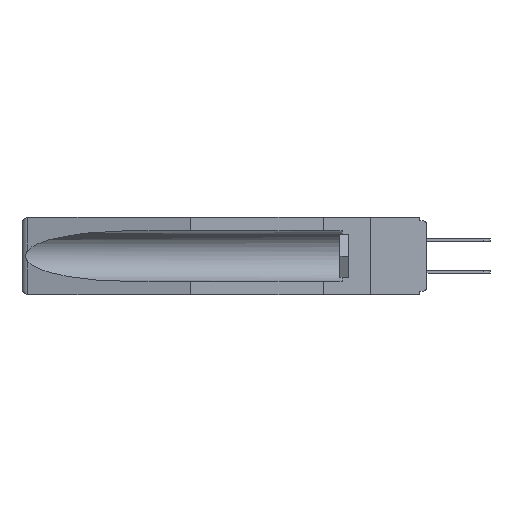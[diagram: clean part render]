
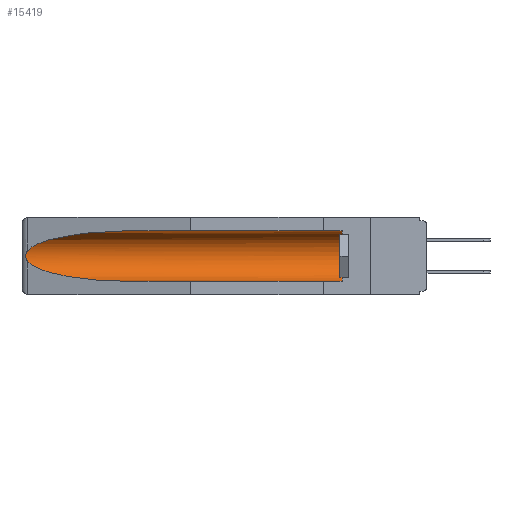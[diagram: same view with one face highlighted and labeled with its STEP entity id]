
A CAD part, left-side view. The second image highlights one B-rep face of the part: STEP entity #15419.
In plain terms, the highlighted cylindrical face has radius 2.857 mm (diameter 5.715 mm), a partial arc.
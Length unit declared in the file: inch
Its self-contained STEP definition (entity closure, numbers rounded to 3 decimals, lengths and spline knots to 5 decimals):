
#138 = CARTESIAN_POINT ( 'NONE',  ( 0.26654, 1.53092, -0.15636 ) ) ;
#239 = VECTOR ( 'NONE', #20241, 39.37008 ) ;
#244 = DIRECTION ( 'NONE',  ( 0., 1., 0. ) ) ;
#271 = CARTESIAN_POINT ( 'NONE',  ( 0.26537, 1.52718, -0.19328 ) ) ;
#353 = CARTESIAN_POINT ( 'NONE',  ( 0.26597, 1.5296, -0.19026 ) ) ;
#610 = ORIENTED_EDGE ( 'NONE', *, *, #13856, .T. ) ;
#1701 = ORIENTED_EDGE ( 'NONE', *, *, #15027, .T. ) ;
#2246 = CARTESIAN_POINT ( 'NONE',  ( 0.155, 1.07973, -0.284 ) ) ;
#2735 = DIRECTION ( 'NONE',  ( 0., 0., 1. ) ) ;
#3331 = VECTOR ( 'NONE', #244, 39.37008 ) ;
#3438 = CARTESIAN_POINT ( 'NONE',  ( 0.2675, 1.53308, -0.17534 ) ) ;
#3753 = ORIENTED_EDGE ( 'NONE', *, *, #21781, .T. ) ;
#3792 = AXIS2_PLACEMENT_3D ( 'NONE', #18318, #21011, #2735 ) ;
#4294 = EDGE_CURVE ( 'NONE', #19812, #9794, #5132, .T. ) ;
#4777 = CARTESIAN_POINT ( 'NONE',  ( 0.21114, 1.30732, -0.284 ) ) ;
#5132 = B_SPLINE_CURVE_WITH_KNOTS ( 'NONE', 3,
 ( #18709, #20573, #138, #10422, #12054, #3438, #15374, #8821, #353, #271 ),
 .UNSPECIFIED., .F., .F.,
 ( 4, 2, 2, 2, 4 ),
 ( 0., 0.00029, 0.00058, 0.00087, 0.00117 ),
 .UNSPECIFIED. ) ;
#5380 = EDGE_CURVE ( 'NONE', #13100, #5696, #18282, .T. ) ;
#5520 = CARTESIAN_POINT ( 'NONE',  ( 0.155, 0.126, -0.059 ) ) ;
#5696 = VERTEX_POINT ( 'NONE', #20296 ) ;
#6453 = AXIS2_PLACEMENT_3D ( 'NONE', #6814, #18595, #10385 ) ;
#6814 = CARTESIAN_POINT ( 'NONE',  ( 0.155, 0.126, -0.1715 ) ) ;
#6970 = CYLINDRICAL_SURFACE ( 'NONE', #3792, 0.1125 ) ;
#7698 = ORIENTED_EDGE ( 'NONE', *, *, #19265, .F. ) ;
#8676 = CARTESIAN_POINT ( 'NONE',  ( 0.26537, 1.52718, -0.19328 ) ) ;
#8821 = CARTESIAN_POINT ( 'NONE',  ( 0.26655, 1.53094, -0.18657 ) ) ;
#8995 = CARTESIAN_POINT ( 'NONE',  ( 0.26537, 1.52718, -0.14972 ) ) ;
#9185 = CARTESIAN_POINT ( 'NONE',  ( 0.26537, 1.52718, -0.14972 ) ) ;
#9591 = CARTESIAN_POINT ( 'NONE',  ( 0.155, 1.07973, -0.284 ) ) ;
#9794 = VERTEX_POINT ( 'NONE', #8676 ) ;
#9878 = VERTEX_POINT ( 'NONE', #2246 ) ;
#10385 = DIRECTION ( 'NONE',  ( 0., 0., 1. ) ) ;
#10422 = CARTESIAN_POINT ( 'NONE',  ( 0.2673, 1.5327, -0.16383 ) ) ;
#10460 = CARTESIAN_POINT ( 'NONE',  ( 0.155, -0.30754, -0.284 ) ) ;
#11533 = CARTESIAN_POINT ( 'NONE',  ( 0.26537, 1.52718, -0.19328 ) ) ;
#12054 = CARTESIAN_POINT ( 'NONE',  ( 0.2675, 1.53308, -0.16763 ) ) ;
#12168 = CARTESIAN_POINT ( 'NONE',  ( 0.21114, 1.30732, -0.059 ) ) ;
#13100 = VERTEX_POINT ( 'NONE', #5520 ) ;
#13334 = CARTESIAN_POINT ( 'NONE',  ( 0.155, -0.30754, -0.059 ) ) ;
#13683 = ORIENTED_EDGE ( 'NONE', *, *, #5380, .T. ) ;
#13729 = EDGE_LOOP ( 'NONE', ( #1701, #15863, #3753, #7698, #610, #13683 ) ) ;
#13856 = EDGE_CURVE ( 'NONE', #19405, #13100, #14693, .T. ) ;
#14103 = FACE_OUTER_BOUND ( 'NONE', #13729, .T. ) ;
#14693 = CIRCLE ( 'NONE', #6453, 0.1125 ) ;
#14937 = CARTESIAN_POINT ( 'NONE',  ( 0.25451, 1.48313, -0.24835 ) ) ;
#15027 = EDGE_CURVE ( 'NONE', #5696, #19812, #21580, .T. ) ;
#15374 = CARTESIAN_POINT ( 'NONE',  ( 0.2673, 1.53269, -0.17917 ) ) ;
#15419 = ADVANCED_FACE ( 'NONE', ( #14103 ), #6970, .F. ) ;
#15626 = CARTESIAN_POINT ( 'NONE',  ( 0.25451, 1.48313, -0.09465 ) ) ;
#15751 = CARTESIAN_POINT ( 'NONE',  ( 0.155, 1.07973, -0.059 ) ) ;
#15863 = ORIENTED_EDGE ( 'NONE', *, *, #4294, .T. ) ;
#18182 = CARTESIAN_POINT ( 'NONE',  ( 0.155, 0.126, -0.284 ) ) ;
#18282 = LINE ( 'NONE', #13334, #239 ) ;
#18318 = CARTESIAN_POINT ( 'NONE',  ( 0.155, -0.30754, -0.1715 ) ) ;
#18595 = DIRECTION ( 'NONE',  ( 0., -1., 0. ) ) ;
#18709 = CARTESIAN_POINT ( 'NONE',  ( 0.26537, 1.52718, -0.14972 ) ) ;
#19257 =( BOUNDED_CURVE ( )  B_SPLINE_CURVE ( 3, ( #11533, #14937, #4777, #9591 ),
 .UNSPECIFIED., .F., .F. ) 
 B_SPLINE_CURVE_WITH_KNOTS ( ( 4, 4 ),
 ( 0.1948, 1.5708 ),
 .UNSPECIFIED. ) 
 CURVE ( )  GEOMETRIC_REPRESENTATION_ITEM ( )  RATIONAL_B_SPLINE_CURVE ( ( 1., 0.848, 0.848, 1. ) ) 
 REPRESENTATION_ITEM ( '' )  );
#19265 = EDGE_CURVE ( 'NONE', #19405, #9878, #20850, .T. ) ;
#19405 = VERTEX_POINT ( 'NONE', #18182 ) ;
#19812 = VERTEX_POINT ( 'NONE', #9185 ) ;
#20241 = DIRECTION ( 'NONE',  ( 0., 1., 0. ) ) ;
#20296 = CARTESIAN_POINT ( 'NONE',  ( 0.155, 1.07973, -0.059 ) ) ;
#20573 = CARTESIAN_POINT ( 'NONE',  ( 0.26597, 1.52961, -0.15275 ) ) ;
#20850 = LINE ( 'NONE', #10460, #3331 ) ;
#21011 = DIRECTION ( 'NONE',  ( 0., 1., 0. ) ) ;
#21580 =( BOUNDED_CURVE ( )  B_SPLINE_CURVE ( 3, ( #15751, #12168, #15626, #8995 ),
 .UNSPECIFIED., .F., .F. ) 
 B_SPLINE_CURVE_WITH_KNOTS ( ( 4, 4 ),
 ( 4.71239, 6.08839 ),
 .UNSPECIFIED. ) 
 CURVE ( )  GEOMETRIC_REPRESENTATION_ITEM ( )  RATIONAL_B_SPLINE_CURVE ( ( 1., 0.848, 0.848, 1. ) ) 
 REPRESENTATION_ITEM ( '' )  );
#21781 = EDGE_CURVE ( 'NONE', #9794, #9878, #19257, .T. ) ;
